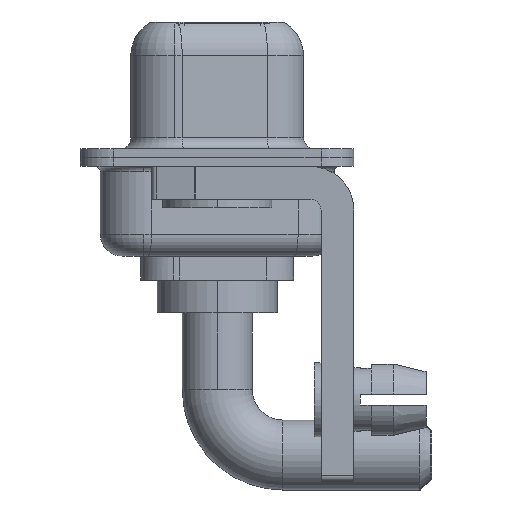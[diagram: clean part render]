
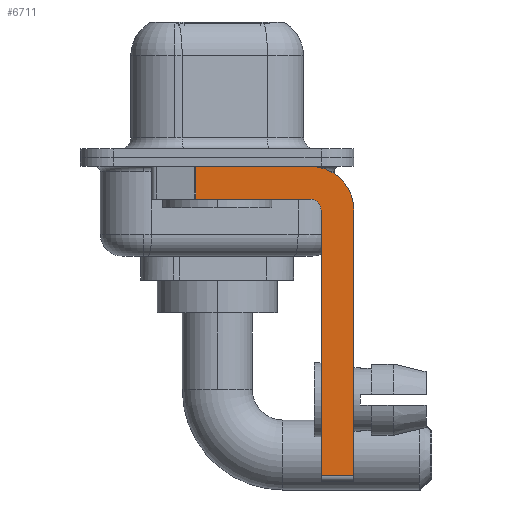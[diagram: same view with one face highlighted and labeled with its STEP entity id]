
A CAD part, left-side view. The second image highlights one B-rep face of the part: STEP entity #6711.
In plain terms, the highlighted planar face has unit normal (-1, 0, 0).
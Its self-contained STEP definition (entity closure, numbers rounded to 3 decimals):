
#86 = ORIENTED_EDGE ( 'NONE', *, *, #7382, .T. ) ;
#93 = DIRECTION ( 'NONE',  ( 0., 1., 0. ) ) ;
#246 = LINE ( 'NONE', #3828, #15494 ) ;
#293 = CARTESIAN_POINT ( 'NONE',  ( -2.9, -4.25, -14.55 ) ) ;
#381 = DIRECTION ( 'NONE',  ( 0., -1., 0. ) ) ;
#1080 = VECTOR ( 'NONE', #1246, 1000. ) ;
#1246 = DIRECTION ( 'NONE',  ( 0., 0., -1. ) ) ;
#1308 = CARTESIAN_POINT ( 'NONE',  ( -2.9, -4.75, -14.55 ) ) ;
#1515 = EDGE_LOOP ( 'NONE', ( #4668, #86, #13773, #4365, #15978, #3267, #5779, #6413 ) ) ;
#1689 = DIRECTION ( 'NONE',  ( 1., 0., 0. ) ) ;
#2041 = CARTESIAN_POINT ( 'NONE',  ( -2.9, 0.978, -1.9 ) ) ;
#2356 = CARTESIAN_POINT ( 'NONE',  ( -2.9, -6.25, -14.55 ) ) ;
#2685 = CARTESIAN_POINT ( 'NONE',  ( -2.9, -6.25, -2.4 ) ) ;
#2751 = CARTESIAN_POINT ( 'NONE',  ( -2.9, 3., -0.4 ) ) ;
#2922 = LINE ( 'NONE', #7936, #9686 ) ;
#3136 = VECTOR ( 'NONE', #381, 1000. ) ;
#3267 = ORIENTED_EDGE ( 'NONE', *, *, #4171, .T. ) ;
#3362 = AXIS2_PLACEMENT_3D ( 'NONE', #6958, #8193, #13356 ) ;
#3802 = CARTESIAN_POINT ( 'NONE',  ( -2.9, -4.25, -1.9 ) ) ;
#3828 = CARTESIAN_POINT ( 'NONE',  ( -2.9, -4.25, -1.9 ) ) ;
#3929 = VECTOR ( 'NONE', #7758, 1000. ) ;
#4171 = EDGE_CURVE ( 'NONE', #8376, #13809, #7805, .T. ) ;
#4224 = DIRECTION ( 'NONE',  ( 0., 0., -1. ) ) ;
#4365 = ORIENTED_EDGE ( 'NONE', *, *, #8196, .F. ) ;
#4482 = CARTESIAN_POINT ( 'NONE',  ( -2.9, -4.25, -2.4 ) ) ;
#4485 = EDGE_CURVE ( 'NONE', #15042, #13809, #7463, .T. ) ;
#4668 = ORIENTED_EDGE ( 'NONE', *, *, #6798, .F. ) ;
#5299 = LINE ( 'NONE', #2751, #3929 ) ;
#5446 = PLANE ( 'NONE',  #10723 ) ;
#5779 = ORIENTED_EDGE ( 'NONE', *, *, #4485, .F. ) ;
#6413 = ORIENTED_EDGE ( 'NONE', *, *, #6545, .F. ) ;
#6545 = EDGE_CURVE ( 'NONE', #14669, #15042, #15186, .T. ) ;
#6711 = ADVANCED_FACE ( 'NONE', ( #15462 ), #5446, .F. ) ;
#6798 = EDGE_CURVE ( 'NONE', #9884, #14669, #5299, .T. ) ;
#6958 = CARTESIAN_POINT ( 'NONE',  ( -2.9, -4.25, -2.4 ) ) ;
#7382 = EDGE_CURVE ( 'NONE', #9884, #13241, #2922, .T. ) ;
#7463 = LINE ( 'NONE', #12467, #1080 ) ;
#7758 = DIRECTION ( 'NONE',  ( 0., -1., 0. ) ) ;
#7805 = LINE ( 'NONE', #293, #3136 ) ;
#7936 = CARTESIAN_POINT ( 'NONE',  ( -2.9, 0.978, -1.9 ) ) ;
#8193 = DIRECTION ( 'NONE',  ( -1., 0., 0. ) ) ;
#8196 = EDGE_CURVE ( 'NONE', #15621, #9902, #8622, .T. ) ;
#8376 = VERTEX_POINT ( 'NONE', #1308 ) ;
#8442 = DIRECTION ( 'NONE',  ( 0., 0., 1. ) ) ;
#8622 = CIRCLE ( 'NONE', #3362, 0.5 ) ;
#8696 = VECTOR ( 'NONE', #8442, 1000. ) ;
#9408 = AXIS2_PLACEMENT_3D ( 'NONE', #4482, #9477, #14497 ) ;
#9477 = DIRECTION ( 'NONE',  ( 1., 0., 0. ) ) ;
#9686 = VECTOR ( 'NONE', #15475, 1000. ) ;
#9884 = VERTEX_POINT ( 'NONE', #12394 ) ;
#9902 = VERTEX_POINT ( 'NONE', #3802 ) ;
#10449 = CARTESIAN_POINT ( 'NONE',  ( -2.9, -4.25, -2.4 ) ) ;
#10723 = AXIS2_PLACEMENT_3D ( 'NONE', #10449, #1689, #4224 ) ;
#12394 = CARTESIAN_POINT ( 'NONE',  ( -2.9, 0.978, -0.4 ) ) ;
#12467 = CARTESIAN_POINT ( 'NONE',  ( -2.9, -6.25, -2.4 ) ) ;
#13241 = VERTEX_POINT ( 'NONE', #2041 ) ;
#13356 = DIRECTION ( 'NONE',  ( 0., 0., 1. ) ) ;
#13615 = CARTESIAN_POINT ( 'NONE',  ( -2.9, -4.75, -14.8 ) ) ;
#13773 = ORIENTED_EDGE ( 'NONE', *, *, #13909, .F. ) ;
#13809 = VERTEX_POINT ( 'NONE', #2356 ) ;
#13909 = EDGE_CURVE ( 'NONE', #9902, #13241, #246, .T. ) ;
#14325 = EDGE_CURVE ( 'NONE', #8376, #15621, #15014, .T. ) ;
#14497 = DIRECTION ( 'NONE',  ( 0., 0., -1. ) ) ;
#14506 = CARTESIAN_POINT ( 'NONE',  ( -2.9, -4.25, -0.4 ) ) ;
#14669 = VERTEX_POINT ( 'NONE', #14506 ) ;
#15014 = LINE ( 'NONE', #13615, #8696 ) ;
#15042 = VERTEX_POINT ( 'NONE', #2685 ) ;
#15186 = CIRCLE ( 'NONE', #9408, 2. ) ;
#15451 = CARTESIAN_POINT ( 'NONE',  ( -2.9, -4.75, -2.4 ) ) ;
#15462 = FACE_OUTER_BOUND ( 'NONE', #1515, .T. ) ;
#15475 = DIRECTION ( 'NONE',  ( 0., 0., -1. ) ) ;
#15494 = VECTOR ( 'NONE', #93, 1000. ) ;
#15621 = VERTEX_POINT ( 'NONE', #15451 ) ;
#15978 = ORIENTED_EDGE ( 'NONE', *, *, #14325, .F. ) ;
